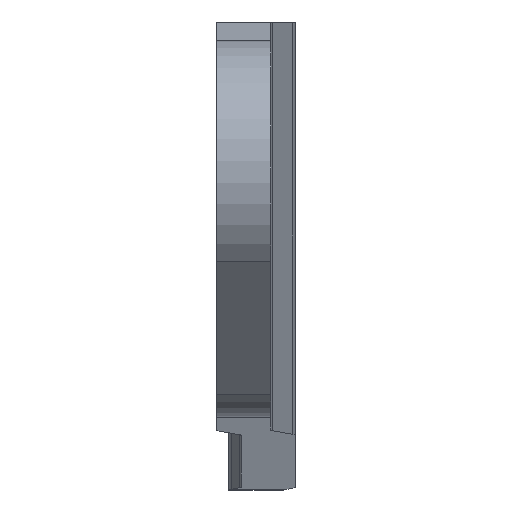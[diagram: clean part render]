
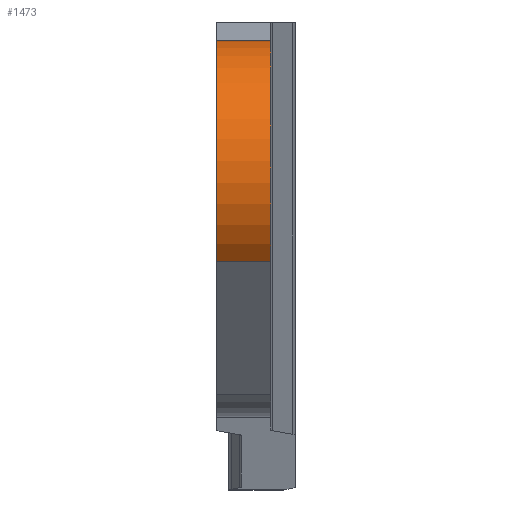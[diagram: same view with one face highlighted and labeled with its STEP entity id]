
A CAD part, top view. The second image highlights one B-rep face of the part: STEP entity #1473.
In plain terms, the highlighted cylindrical face has radius 5.563 mm (diameter 11.125 mm), a partial arc.
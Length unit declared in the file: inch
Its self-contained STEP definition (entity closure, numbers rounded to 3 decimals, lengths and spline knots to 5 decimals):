
#108=FACE_OUTER_BOUND('',#194,.T.);
#194=EDGE_LOOP('',(#1110,#1111,#1112,#1113));
#267=CIRCLE('',#1564,0.219);
#272=CIRCLE('',#1574,0.219);
#404=LINE('',#3414,#507);
#408=LINE('',#3423,#511);
#507=VECTOR('',#1778,0.3937);
#511=VECTOR('',#1788,0.3937);
#655=VERTEX_POINT('',#3388);
#656=VERTEX_POINT('',#3390);
#664=VERTEX_POINT('',#3411);
#667=VERTEX_POINT('',#3421);
#821=EDGE_CURVE('',#655,#656,#267,.T.);
#832=EDGE_CURVE('',#655,#664,#404,.T.);
#836=EDGE_CURVE('',#667,#664,#272,.T.);
#837=EDGE_CURVE('',#656,#667,#408,.T.);
#1110=ORIENTED_EDGE('',*,*,#836,.F.);
#1111=ORIENTED_EDGE('',*,*,#837,.F.);
#1112=ORIENTED_EDGE('',*,*,#821,.F.);
#1113=ORIENTED_EDGE('',*,*,#832,.T.);
#1420=CYLINDRICAL_SURFACE('',#1573,0.219);
#1473=ADVANCED_FACE('',(#108),#1420,.T.);
#1564=AXIS2_PLACEMENT_3D('',#3391,#1756,#1757);
#1573=AXIS2_PLACEMENT_3D('',#3420,#1784,#1785);
#1574=AXIS2_PLACEMENT_3D('',#3422,#1786,#1787);
#1756=DIRECTION('center_axis',(1.,0.,0.));
#1757=DIRECTION('ref_axis',(0.,1.,0.));
#1778=DIRECTION('',(-1.,0.,0.));
#1784=DIRECTION('center_axis',(-1.,0.,0.));
#1785=DIRECTION('ref_axis',(0.,1.,0.));
#1786=DIRECTION('center_axis',(-1.,0.,0.));
#1787=DIRECTION('ref_axis',(0.,1.,0.));
#1788=DIRECTION('',(-1.,0.,0.));
#3388=CARTESIAN_POINT('',(0.55475,-0.031,3.265));
#3390=CARTESIAN_POINT('',(0.55475,-0.39606,3.42818));
#3391=CARTESIAN_POINT('Origin',(0.55475,-0.25,3.265));
#3411=CARTESIAN_POINT('',(0.46475,-0.031,3.265));
#3414=CARTESIAN_POINT('',(0.59519,-0.031,3.265));
#3420=CARTESIAN_POINT('Origin',(0.59519,-0.25,3.265));
#3421=CARTESIAN_POINT('',(0.46475,-0.39606,3.42818));
#3422=CARTESIAN_POINT('Origin',(0.46475,-0.25,3.265));
#3423=CARTESIAN_POINT('',(0.59519,-0.39606,3.42818));
